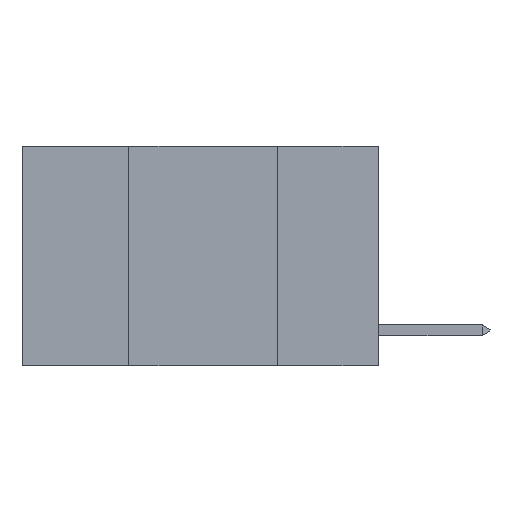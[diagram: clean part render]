
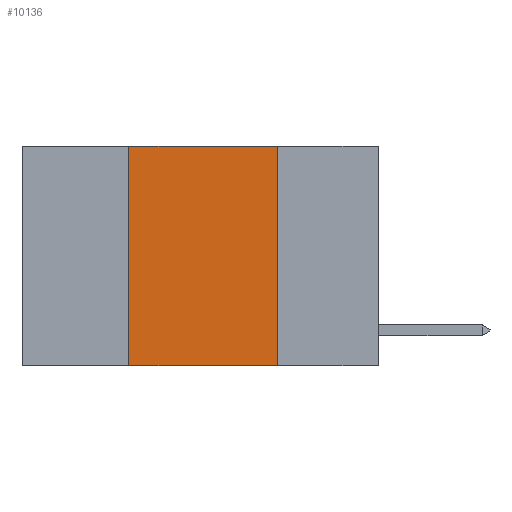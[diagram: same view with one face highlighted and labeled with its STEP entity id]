
A CAD part, left-side view. The second image highlights one B-rep face of the part: STEP entity #10136.
In plain terms, the highlighted planar face has unit normal (-1, 0, 0).
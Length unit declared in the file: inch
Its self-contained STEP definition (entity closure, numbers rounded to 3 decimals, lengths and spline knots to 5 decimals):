
#1104 = VERTEX_POINT ( 'NONE', #6750 ) ;
#1443 = EDGE_CURVE ( 'NONE', #6253, #2857, #20277, .T. ) ;
#1453 = CARTESIAN_POINT ( 'NONE',  ( 0., 0.17, 0. ) ) ;
#2857 = VERTEX_POINT ( 'NONE', #1453 ) ;
#3015 = VERTEX_POINT ( 'NONE', #15837 ) ;
#3870 = ORIENTED_EDGE ( 'NONE', *, *, #16764, .F. ) ;
#4759 = DIRECTION ( 'NONE',  ( 0., -1., 0. ) ) ;
#6253 = VERTEX_POINT ( 'NONE', #18779 ) ;
#6750 = CARTESIAN_POINT ( 'NONE',  ( 0., 0.42, -0.37 ) ) ;
#6794 = DIRECTION ( 'NONE',  ( 0., 0., -1. ) ) ;
#7811 = DIRECTION ( 'NONE',  ( 0., -1., 0. ) ) ;
#7902 = VECTOR ( 'NONE', #4759, 39.37008 ) ;
#8494 = PLANE ( 'NONE',  #8783 ) ;
#8587 = EDGE_CURVE ( 'NONE', #1104, #3015, #14857, .T. ) ;
#8783 = AXIS2_PLACEMENT_3D ( 'NONE', #15440, #22308, #6794 ) ;
#10136 = ADVANCED_FACE ( 'NONE', ( #17138 ), #8494, .F. ) ;
#11656 = CARTESIAN_POINT ( 'NONE',  ( 0., 0.6, 0. ) ) ;
#12268 = ORIENTED_EDGE ( 'NONE', *, *, #18262, .F. ) ;
#12346 = ORIENTED_EDGE ( 'NONE', *, *, #8587, .T. ) ;
#13518 = CARTESIAN_POINT ( 'NONE',  ( 0., 0.17, 0. ) ) ;
#14857 = LINE ( 'NONE', #21732, #15144 ) ;
#15144 = VECTOR ( 'NONE', #7811, 39.37008 ) ;
#15415 = ORIENTED_EDGE ( 'NONE', *, *, #1443, .F. ) ;
#15440 = CARTESIAN_POINT ( 'NONE',  ( 0., 0.6, 0. ) ) ;
#15808 = DIRECTION ( 'NONE',  ( 0., 0., 1. ) ) ;
#15837 = CARTESIAN_POINT ( 'NONE',  ( 0., 0.17, -0.37 ) ) ;
#16764 = EDGE_CURVE ( 'NONE', #2857, #3015, #18840, .T. ) ;
#17138 = FACE_OUTER_BOUND ( 'NONE', #21378, .T. ) ;
#17160 = DIRECTION ( 'NONE',  ( 0., 0., -1. ) ) ;
#18262 = EDGE_CURVE ( 'NONE', #1104, #6253, #19275, .T. ) ;
#18641 = VECTOR ( 'NONE', #17160, 39.37008 ) ;
#18779 = CARTESIAN_POINT ( 'NONE',  ( 0., 0.42, 0. ) ) ;
#18840 = LINE ( 'NONE', #13518, #18641 ) ;
#19275 = LINE ( 'NONE', #19505, #20142 ) ;
#19505 = CARTESIAN_POINT ( 'NONE',  ( 0., 0.42, 0. ) ) ;
#20142 = VECTOR ( 'NONE', #15808, 39.37008 ) ;
#20277 = LINE ( 'NONE', #11656, #7902 ) ;
#21378 = EDGE_LOOP ( 'NONE', ( #3870, #15415, #12268, #12346 ) ) ;
#21732 = CARTESIAN_POINT ( 'NONE',  ( 0., 0.6, -0.37 ) ) ;
#22308 = DIRECTION ( 'NONE',  ( 1., 0., 0. ) ) ;
